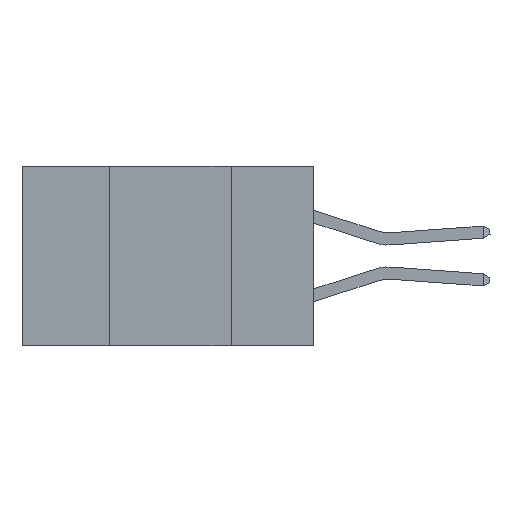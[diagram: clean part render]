
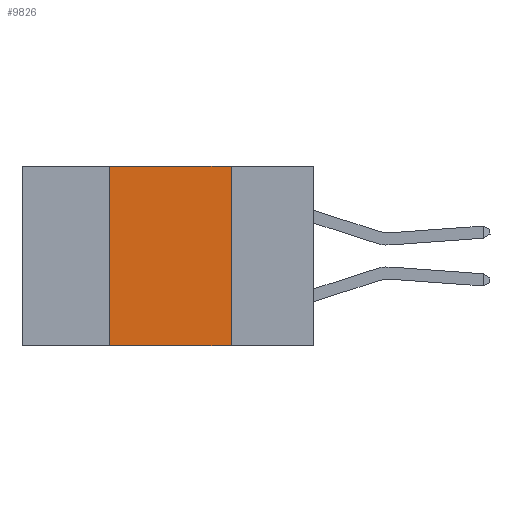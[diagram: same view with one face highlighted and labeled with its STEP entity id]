
A CAD part, left-side view. The second image highlights one B-rep face of the part: STEP entity #9826.
In plain terms, the highlighted planar face has unit normal (-1, 0, 0).
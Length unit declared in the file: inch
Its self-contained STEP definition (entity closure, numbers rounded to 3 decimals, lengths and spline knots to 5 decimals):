
#75 = CARTESIAN_POINT ( 'NONE',  ( 0., 0.6, 0. ) ) ;
#1925 = CARTESIAN_POINT ( 'NONE',  ( 0., 0.42, 0. ) ) ;
#2206 = DIRECTION ( 'NONE',  ( 0., 0., -1. ) ) ;
#2304 = CARTESIAN_POINT ( 'NONE',  ( 0., 0.42, -0.37 ) ) ;
#2639 = EDGE_CURVE ( 'NONE', #8307, #4888, #12604, .T. ) ;
#2953 = ORIENTED_EDGE ( 'NONE', *, *, #10633, .F. ) ;
#3247 = VERTEX_POINT ( 'NONE', #3839 ) ;
#3839 = CARTESIAN_POINT ( 'NONE',  ( 0., 0.42, 0. ) ) ;
#4778 = EDGE_CURVE ( 'NONE', #8307, #3247, #6998, .T. ) ;
#4888 = VERTEX_POINT ( 'NONE', #18282 ) ;
#5117 = CARTESIAN_POINT ( 'NONE',  ( 0., 0.17, 0. ) ) ;
#5155 = ORIENTED_EDGE ( 'NONE', *, *, #17720, .F. ) ;
#5639 = EDGE_LOOP ( 'NONE', ( #5155, #2953, #6702, #5980 ) ) ;
#5980 = ORIENTED_EDGE ( 'NONE', *, *, #2639, .T. ) ;
#6047 = CARTESIAN_POINT ( 'NONE',  ( 0., 0.6, -0.37 ) ) ;
#6702 = ORIENTED_EDGE ( 'NONE', *, *, #4778, .F. ) ;
#6998 = LINE ( 'NONE', #1925, #10905 ) ;
#7729 = VECTOR ( 'NONE', #2206, 39.37008 ) ;
#8307 = VERTEX_POINT ( 'NONE', #2304 ) ;
#8876 = CARTESIAN_POINT ( 'NONE',  ( 0., 0.17, 0. ) ) ;
#9826 = ADVANCED_FACE ( 'NONE', ( #20047 ), #14999, .F. ) ;
#10315 = AXIS2_PLACEMENT_3D ( 'NONE', #19613, #13482, #14774 ) ;
#10633 = EDGE_CURVE ( 'NONE', #3247, #14438, #11487, .T. ) ;
#10905 = VECTOR ( 'NONE', #19684, 39.37008 ) ;
#11087 = DIRECTION ( 'NONE',  ( 0., -1., 0. ) ) ;
#11487 = LINE ( 'NONE', #75, #16534 ) ;
#12604 = LINE ( 'NONE', #6047, #14553 ) ;
#13008 = DIRECTION ( 'NONE',  ( 0., -1., 0. ) ) ;
#13482 = DIRECTION ( 'NONE',  ( 1., 0., 0. ) ) ;
#14438 = VERTEX_POINT ( 'NONE', #5117 ) ;
#14553 = VECTOR ( 'NONE', #11087, 39.37008 ) ;
#14774 = DIRECTION ( 'NONE',  ( 0., 0., -1. ) ) ;
#14999 = PLANE ( 'NONE',  #10315 ) ;
#16534 = VECTOR ( 'NONE', #13008, 39.37008 ) ;
#17720 = EDGE_CURVE ( 'NONE', #14438, #4888, #20182, .T. ) ;
#18282 = CARTESIAN_POINT ( 'NONE',  ( 0., 0.17, -0.37 ) ) ;
#19613 = CARTESIAN_POINT ( 'NONE',  ( 0., 0.6, 0. ) ) ;
#19684 = DIRECTION ( 'NONE',  ( 0., 0., 1. ) ) ;
#20047 = FACE_OUTER_BOUND ( 'NONE', #5639, .T. ) ;
#20182 = LINE ( 'NONE', #8876, #7729 ) ;
